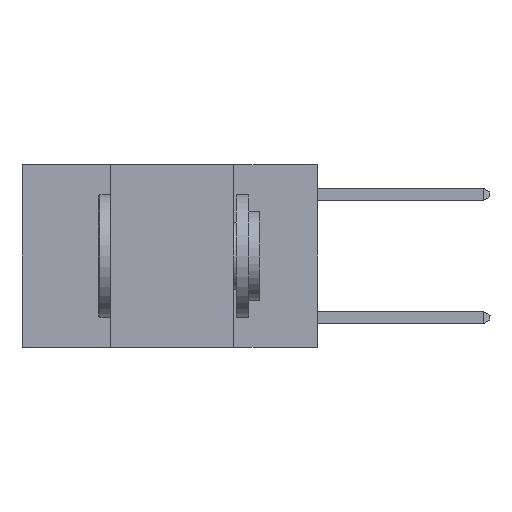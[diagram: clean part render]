
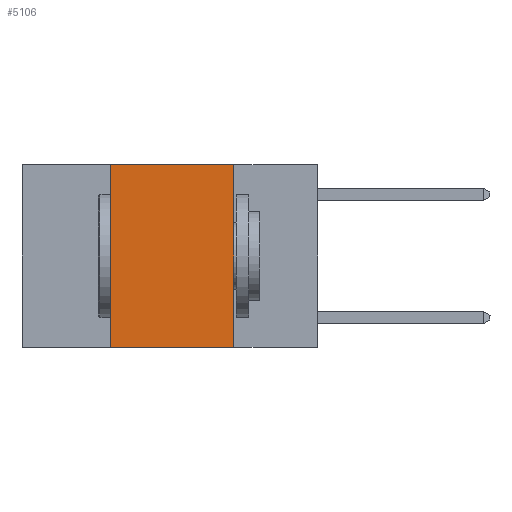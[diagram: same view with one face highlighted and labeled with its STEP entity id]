
A CAD part, left-side view. The second image highlights one B-rep face of the part: STEP entity #5106.
In plain terms, the highlighted planar face has unit normal (-1, 0, 0).
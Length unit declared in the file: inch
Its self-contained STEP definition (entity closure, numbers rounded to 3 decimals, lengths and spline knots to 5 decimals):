
#1877 = CARTESIAN_POINT ( 'NONE',  ( 0., 0.6, 0. ) ) ;
#2101 = LINE ( 'NONE', #25598, #23321 ) ;
#2246 = DIRECTION ( 'NONE',  ( 0., -1., 0. ) ) ;
#2671 = EDGE_CURVE ( 'NONE', #24507, #21654, #2101, .T. ) ;
#3295 = LINE ( 'NONE', #16679, #25131 ) ;
#3989 = DIRECTION ( 'NONE',  ( 1., 0., 0. ) ) ;
#5106 = ADVANCED_FACE ( 'NONE', ( #13845 ), #24464, .F. ) ;
#5132 = DIRECTION ( 'NONE',  ( 0., 0., 1. ) ) ;
#5826 = ORIENTED_EDGE ( 'NONE', *, *, #2671, .F. ) ;
#7382 = LINE ( 'NONE', #10819, #17057 ) ;
#9138 = LINE ( 'NONE', #19321, #14610 ) ;
#9654 = EDGE_CURVE ( 'NONE', #24507, #20369, #7382, .T. ) ;
#10819 = CARTESIAN_POINT ( 'NONE',  ( 0., 0.6, -0.37 ) ) ;
#10891 = CARTESIAN_POINT ( 'NONE',  ( 0., 0.42, 0. ) ) ;
#11977 = CARTESIAN_POINT ( 'NONE',  ( 0., 0.42, -0.37 ) ) ;
#12812 = CARTESIAN_POINT ( 'NONE',  ( 0., 0.17, -0.37 ) ) ;
#13627 = AXIS2_PLACEMENT_3D ( 'NONE', #1877, #3989, #18380 ) ;
#13845 = FACE_OUTER_BOUND ( 'NONE', #19369, .T. ) ;
#14469 = ORIENTED_EDGE ( 'NONE', *, *, #9654, .T. ) ;
#14610 = VECTOR ( 'NONE', #23417, 39.37008 ) ;
#16679 = CARTESIAN_POINT ( 'NONE',  ( 0., 0.6, 0. ) ) ;
#17057 = VECTOR ( 'NONE', #21110, 39.37008 ) ;
#17135 = EDGE_CURVE ( 'NONE', #19342, #20369, #9138, .T. ) ;
#18053 = ORIENTED_EDGE ( 'NONE', *, *, #17135, .F. ) ;
#18296 = EDGE_CURVE ( 'NONE', #21654, #19342, #3295, .T. ) ;
#18380 = DIRECTION ( 'NONE',  ( 0., 0., -1. ) ) ;
#19321 = CARTESIAN_POINT ( 'NONE',  ( 0., 0.17, 0. ) ) ;
#19342 = VERTEX_POINT ( 'NONE', #24008 ) ;
#19369 = EDGE_LOOP ( 'NONE', ( #18053, #25933, #5826, #14469 ) ) ;
#20369 = VERTEX_POINT ( 'NONE', #12812 ) ;
#21110 = DIRECTION ( 'NONE',  ( 0., -1., 0. ) ) ;
#21654 = VERTEX_POINT ( 'NONE', #10891 ) ;
#23321 = VECTOR ( 'NONE', #5132, 39.37008 ) ;
#23417 = DIRECTION ( 'NONE',  ( 0., 0., -1. ) ) ;
#24008 = CARTESIAN_POINT ( 'NONE',  ( 0., 0.17, 0. ) ) ;
#24464 = PLANE ( 'NONE',  #13627 ) ;
#24507 = VERTEX_POINT ( 'NONE', #11977 ) ;
#25131 = VECTOR ( 'NONE', #2246, 39.37008 ) ;
#25598 = CARTESIAN_POINT ( 'NONE',  ( 0., 0.42, 0. ) ) ;
#25933 = ORIENTED_EDGE ( 'NONE', *, *, #18296, .F. ) ;
